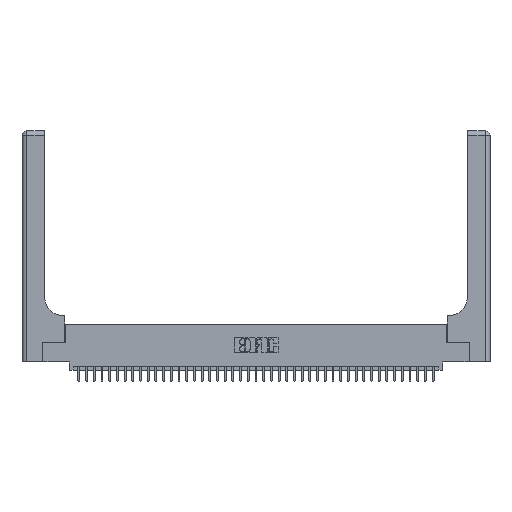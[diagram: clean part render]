
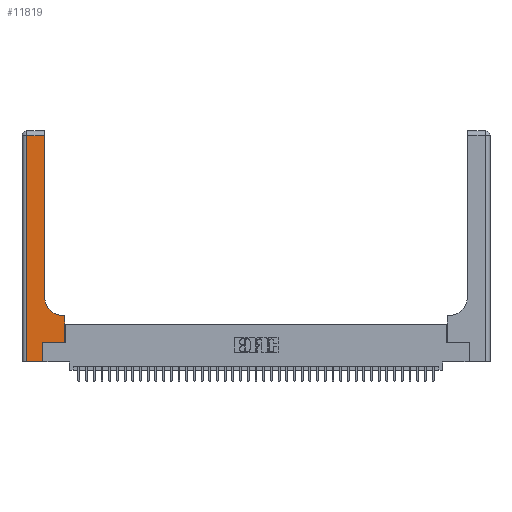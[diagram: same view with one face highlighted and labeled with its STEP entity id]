
A CAD part, top view. The second image highlights one B-rep face of the part: STEP entity #11819.
In plain terms, the highlighted planar face has unit normal (0, 0, 1).
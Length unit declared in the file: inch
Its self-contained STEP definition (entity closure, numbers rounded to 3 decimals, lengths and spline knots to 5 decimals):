
#556 = EDGE_CURVE ( 'NONE', #6878, #34960, #31248, .T. ) ;
#872 = VECTOR ( 'NONE', #6121, 39.37008 ) ;
#1793 = VERTEX_POINT ( 'NONE', #21890 ) ;
#2451 = EDGE_CURVE ( 'NONE', #13719, #1793, #26987, .T. ) ;
#3107 = ORIENTED_EDGE ( 'NONE', *, *, #21384, .T. ) ;
#3765 = VECTOR ( 'NONE', #35877, 39.37008 ) ;
#3776 = VERTEX_POINT ( 'NONE', #28236 ) ;
#4617 = ORIENTED_EDGE ( 'NONE', *, *, #35381, .T. ) ;
#5887 = VERTEX_POINT ( 'NONE', #29938 ) ;
#6121 = DIRECTION ( 'NONE',  ( 0., 1., 0. ) ) ;
#6604 = CARTESIAN_POINT ( 'NONE',  ( 0.5415, 0.6, 0.37 ) ) ;
#6768 = LINE ( 'NONE', #37407, #38921 ) ;
#6878 = VERTEX_POINT ( 'NONE', #6604 ) ;
#7458 = VECTOR ( 'NONE', #12063, 39.37008 ) ;
#7750 = EDGE_LOOP ( 'NONE', ( #28163, #38751, #16080, #24648, #3107, #13608, #8105, #4617, #38791 ) ) ;
#8105 = ORIENTED_EDGE ( 'NONE', *, *, #16328, .T. ) ;
#8114 = EDGE_CURVE ( 'NONE', #34960, #10008, #10403, .T. ) ;
#8569 = CARTESIAN_POINT ( 'NONE',  ( 0.269, 0.25, 0.37 ) ) ;
#8988 = CARTESIAN_POINT ( 'NONE',  ( 0., 3., 0.37 ) ) ;
#9425 = VECTOR ( 'NONE', #29531, 39.37008 ) ;
#9831 = EDGE_CURVE ( 'NONE', #1793, #39374, #6768, .T. ) ;
#10008 = VERTEX_POINT ( 'NONE', #38397 ) ;
#10403 = LINE ( 'NONE', #22080, #872 ) ;
#10430 = LINE ( 'NONE', #16601, #9425 ) ;
#10470 = LINE ( 'NONE', #31990, #20993 ) ;
#11819 = ADVANCED_FACE ( 'NONE', ( #26145 ), #18506, .F. ) ;
#12063 = DIRECTION ( 'NONE',  ( 0., -1., 0. ) ) ;
#12240 = DIRECTION ( 'NONE',  ( 0., 0., -1. ) ) ;
#12293 = LINE ( 'NONE', #16579, #3765 ) ;
#13608 = ORIENTED_EDGE ( 'NONE', *, *, #21443, .T. ) ;
#13719 = VERTEX_POINT ( 'NONE', #15125 ) ;
#13992 = LINE ( 'NONE', #28969, #24540 ) ;
#14926 = DIRECTION ( 'NONE',  ( 0., 0., -1. ) ) ;
#15125 = CARTESIAN_POINT ( 'NONE',  ( 0.06, 2.94, 0.37 ) ) ;
#15251 = CARTESIAN_POINT ( 'NONE',  ( 0.06, 3., 0.37 ) ) ;
#16080 = ORIENTED_EDGE ( 'NONE', *, *, #2451, .T. ) ;
#16328 = EDGE_CURVE ( 'NONE', #5887, #3776, #10430, .T. ) ;
#16579 = CARTESIAN_POINT ( 'NONE',  ( 0.2915, 0.6, 0.37 ) ) ;
#16601 = CARTESIAN_POINT ( 'NONE',  ( 0.5585, 0.25, 0.37 ) ) ;
#18506 = PLANE ( 'NONE',  #31470 ) ;
#18899 = CARTESIAN_POINT ( 'NONE',  ( 0.269, 0., 0.37 ) ) ;
#19877 = AXIS2_PLACEMENT_3D ( 'NONE', #34230, #14926, #37436 ) ;
#20020 = CARTESIAN_POINT ( 'NONE',  ( 0.269, 0., 0.37 ) ) ;
#20993 = VECTOR ( 'NONE', #35238, 39.37008 ) ;
#21384 = EDGE_CURVE ( 'NONE', #39374, #23328, #28542, .T. ) ;
#21443 = EDGE_CURVE ( 'NONE', #23328, #5887, #10470, .T. ) ;
#21513 = DIRECTION ( 'NONE',  ( 1., 0., 0. ) ) ;
#21890 = CARTESIAN_POINT ( 'NONE',  ( 0.06, 0., 0.37 ) ) ;
#22014 = VECTOR ( 'NONE', #41387, 39.37008 ) ;
#22080 = CARTESIAN_POINT ( 'NONE',  ( 0.2915, 3., 0.37 ) ) ;
#23328 = VERTEX_POINT ( 'NONE', #8569 ) ;
#24335 = CARTESIAN_POINT ( 'NONE',  ( 0.2915, 0.85, 0.37 ) ) ;
#24540 = VECTOR ( 'NONE', #38674, 39.37008 ) ;
#24648 = ORIENTED_EDGE ( 'NONE', *, *, #9831, .T. ) ;
#26145 = FACE_OUTER_BOUND ( 'NONE', #7750, .T. ) ;
#26987 = LINE ( 'NONE', #15251, #7458 ) ;
#27215 = EDGE_CURVE ( 'NONE', #10008, #13719, #13992, .T. ) ;
#28163 = ORIENTED_EDGE ( 'NONE', *, *, #8114, .T. ) ;
#28236 = CARTESIAN_POINT ( 'NONE',  ( 0.5585, 0.6, 0.37 ) ) ;
#28542 = LINE ( 'NONE', #18899, #22014 ) ;
#28969 = CARTESIAN_POINT ( 'NONE',  ( 0., 2.94, 0.37 ) ) ;
#29531 = DIRECTION ( 'NONE',  ( 0., 1., 0. ) ) ;
#29938 = CARTESIAN_POINT ( 'NONE',  ( 0.5585, 0.25, 0.37 ) ) ;
#31248 = CIRCLE ( 'NONE', #19877, 0.25 ) ;
#31470 = AXIS2_PLACEMENT_3D ( 'NONE', #8988, #12240, #34714 ) ;
#31990 = CARTESIAN_POINT ( 'NONE',  ( 0.269, 0.25, 0.37 ) ) ;
#34230 = CARTESIAN_POINT ( 'NONE',  ( 0.5415, 0.85, 0.37 ) ) ;
#34714 = DIRECTION ( 'NONE',  ( -1., 0., 0. ) ) ;
#34960 = VERTEX_POINT ( 'NONE', #24335 ) ;
#35238 = DIRECTION ( 'NONE',  ( 1., 0., 0. ) ) ;
#35381 = EDGE_CURVE ( 'NONE', #3776, #6878, #12293, .T. ) ;
#35877 = DIRECTION ( 'NONE',  ( -1., 0., 0. ) ) ;
#37407 = CARTESIAN_POINT ( 'NONE',  ( 0., 0., 0.37 ) ) ;
#37436 = DIRECTION ( 'NONE',  ( 1., 0., 0. ) ) ;
#38397 = CARTESIAN_POINT ( 'NONE',  ( 0.2915, 2.94, 0.37 ) ) ;
#38674 = DIRECTION ( 'NONE',  ( -1., 0., 0. ) ) ;
#38751 = ORIENTED_EDGE ( 'NONE', *, *, #27215, .T. ) ;
#38791 = ORIENTED_EDGE ( 'NONE', *, *, #556, .T. ) ;
#38921 = VECTOR ( 'NONE', #21513, 39.37008 ) ;
#39374 = VERTEX_POINT ( 'NONE', #20020 ) ;
#41387 = DIRECTION ( 'NONE',  ( 0., 1., 0. ) ) ;
